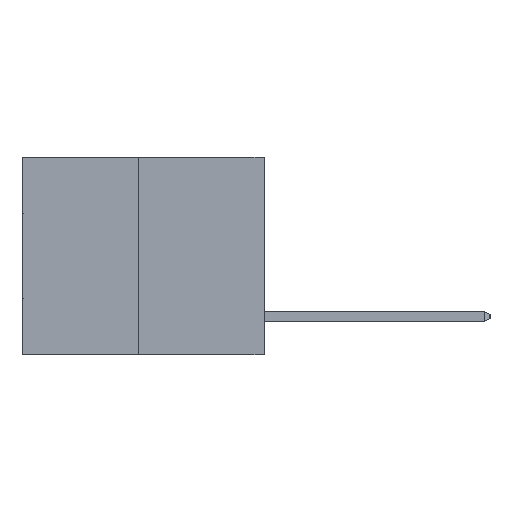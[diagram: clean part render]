
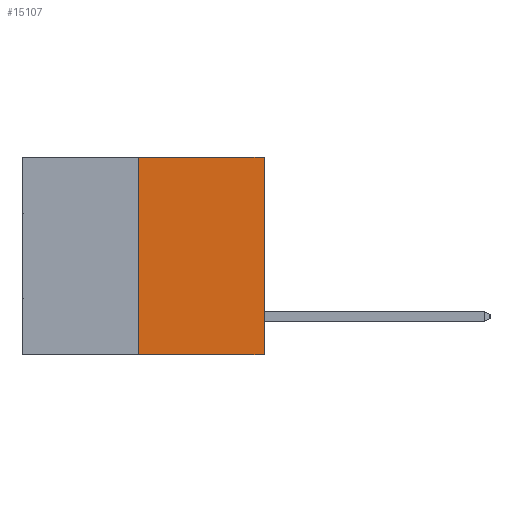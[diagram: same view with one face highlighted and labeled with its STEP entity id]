
A CAD part, left-side view. The second image highlights one B-rep face of the part: STEP entity #15107.
In plain terms, the highlighted planar face has unit normal (-1, 0, 0).
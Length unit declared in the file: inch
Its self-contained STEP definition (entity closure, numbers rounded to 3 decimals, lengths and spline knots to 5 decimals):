
#651 = PLANE ( 'NONE',  #31363 ) ;
#1686 = ORIENTED_EDGE ( 'NONE', *, *, #22341, .F. ) ;
#2118 = EDGE_LOOP ( 'NONE', ( #4725, #9781, #24086, #1686 ) ) ;
#4725 = ORIENTED_EDGE ( 'NONE', *, *, #5429, .F. ) ;
#5429 = EDGE_CURVE ( 'NONE', #13129, #26644, #22486, .T. ) ;
#5911 = CARTESIAN_POINT ( 'NONE',  ( 0., 0., 0. ) ) ;
#6008 = FACE_OUTER_BOUND ( 'NONE', #2118, .T. ) ;
#6513 = CARTESIAN_POINT ( 'NONE',  ( 0., 0., 0. ) ) ;
#9273 = EDGE_CURVE ( 'NONE', #20837, #28307, #29764, .T. ) ;
#9781 = ORIENTED_EDGE ( 'NONE', *, *, #31249, .T. ) ;
#13129 = VERTEX_POINT ( 'NONE', #26376 ) ;
#13308 = CARTESIAN_POINT ( 'NONE',  ( 0., 0.6, 0. ) ) ;
#13465 = DIRECTION ( 'NONE',  ( 1., 0., 0. ) ) ;
#15107 = ADVANCED_FACE ( 'NONE', ( #6008 ), #651, .F. ) ;
#15119 = DIRECTION ( 'NONE',  ( 0., -1., 0. ) ) ;
#15811 = DIRECTION ( 'NONE',  ( 0., -1., 0. ) ) ;
#16327 = VECTOR ( 'NONE', #27667, 39.37008 ) ;
#17349 = CARTESIAN_POINT ( 'NONE',  ( 0., 0.6, -0.49 ) ) ;
#19854 = VECTOR ( 'NONE', #15811, 39.37008 ) ;
#20266 = CARTESIAN_POINT ( 'NONE',  ( 0., 0.312, -0.49 ) ) ;
#20837 = VERTEX_POINT ( 'NONE', #28579 ) ;
#21315 = VECTOR ( 'NONE', #29988, 39.37008 ) ;
#22341 = EDGE_CURVE ( 'NONE', #26644, #28307, #26397, .T. ) ;
#22486 = LINE ( 'NONE', #20266, #16327 ) ;
#22901 = CARTESIAN_POINT ( 'NONE',  ( 0., 0.312, 0. ) ) ;
#23561 = LINE ( 'NONE', #17349, #27773 ) ;
#24086 = ORIENTED_EDGE ( 'NONE', *, *, #9273, .T. ) ;
#25553 = CARTESIAN_POINT ( 'NONE',  ( 0., 0.6, 0. ) ) ;
#26376 = CARTESIAN_POINT ( 'NONE',  ( 0., 0.312, -0.49 ) ) ;
#26397 = LINE ( 'NONE', #13308, #19854 ) ;
#26644 = VERTEX_POINT ( 'NONE', #22901 ) ;
#27667 = DIRECTION ( 'NONE',  ( 0., 0., 1. ) ) ;
#27773 = VECTOR ( 'NONE', #15119, 39.37008 ) ;
#28307 = VERTEX_POINT ( 'NONE', #5911 ) ;
#28579 = CARTESIAN_POINT ( 'NONE',  ( 0., 0., -0.49 ) ) ;
#29764 = LINE ( 'NONE', #6513, #21315 ) ;
#29988 = DIRECTION ( 'NONE',  ( 0., 0., 1. ) ) ;
#30768 = DIRECTION ( 'NONE',  ( 0., 0., -1. ) ) ;
#31249 = EDGE_CURVE ( 'NONE', #13129, #20837, #23561, .T. ) ;
#31363 = AXIS2_PLACEMENT_3D ( 'NONE', #25553, #13465, #30768 ) ;
